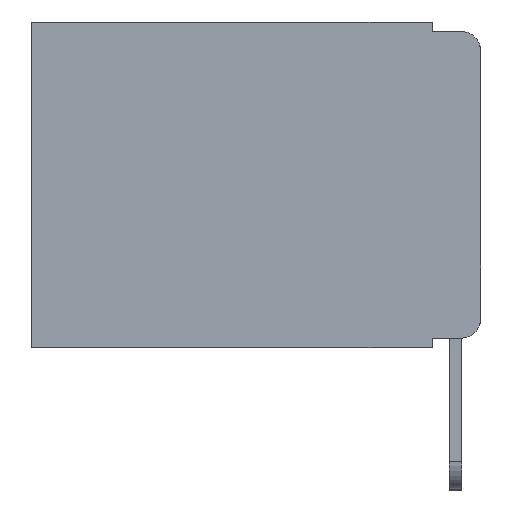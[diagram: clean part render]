
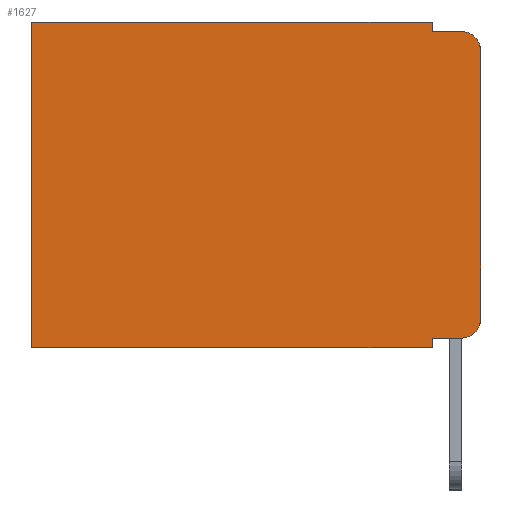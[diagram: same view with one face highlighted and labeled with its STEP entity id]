
A CAD part, left-side view. The second image highlights one B-rep face of the part: STEP entity #1627.
In plain terms, the highlighted planar face has unit normal (-1, 0, 0).
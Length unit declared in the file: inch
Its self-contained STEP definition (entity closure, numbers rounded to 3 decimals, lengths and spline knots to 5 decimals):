
#272 = CIRCLE ( 'NONE', #9551, 0.02 ) ;
#460 = VERTEX_POINT ( 'NONE', #11396 ) ;
#861 = VECTOR ( 'NONE', #10455, 39.37008 ) ;
#1310 = AXIS2_PLACEMENT_3D ( 'NONE', #9073, #3882, #10256 ) ;
#1342 = DIRECTION ( 'NONE',  ( 0., 1., 0. ) ) ;
#1490 = VECTOR ( 'NONE', #3290, 39.37008 ) ;
#1609 = EDGE_CURVE ( 'NONE', #9750, #5757, #6083, .T. ) ;
#1627 = ADVANCED_FACE ( 'NONE', ( #3625 ), #3471, .F. ) ;
#1780 = EDGE_CURVE ( 'NONE', #5310, #5757, #6770, .T. ) ;
#1840 = EDGE_CURVE ( 'NONE', #4678, #5310, #3176, .T. ) ;
#1926 = VERTEX_POINT ( 'NONE', #10651 ) ;
#2858 = VERTEX_POINT ( 'NONE', #3970 ) ;
#2883 = LINE ( 'NONE', #9524, #5368 ) ;
#3152 = DIRECTION ( 'NONE',  ( 0., 1., 0. ) ) ;
#3176 = LINE ( 'NONE', #5163, #7730 ) ;
#3192 = CARTESIAN_POINT ( 'NONE',  ( 0.298, 0.051, 0. ) ) ;
#3243 = EDGE_CURVE ( 'NONE', #6789, #460, #3718, .T. ) ;
#3264 = CARTESIAN_POINT ( 'NONE',  ( 0.298, 0.051, -0.01 ) ) ;
#3290 = DIRECTION ( 'NONE',  ( 0., 0., -1. ) ) ;
#3349 = DIRECTION ( 'NONE',  ( 1., 0., 0. ) ) ;
#3393 = DIRECTION ( 'NONE',  ( 0., 0., -1. ) ) ;
#3471 = PLANE ( 'NONE',  #3967 ) ;
#3625 = FACE_OUTER_BOUND ( 'NONE', #4723, .T. ) ;
#3718 = LINE ( 'NONE', #9774, #8160 ) ;
#3833 = VECTOR ( 'NONE', #3152, 39.37008 ) ;
#3861 = VERTEX_POINT ( 'NONE', #9793 ) ;
#3882 = DIRECTION ( 'NONE',  ( -1., 0., 0. ) ) ;
#3936 = CARTESIAN_POINT ( 'NONE',  ( 0.298, 0., 0. ) ) ;
#3967 = AXIS2_PLACEMENT_3D ( 'NONE', #7719, #3349, #3393 ) ;
#3970 = CARTESIAN_POINT ( 'NONE',  ( 0.298, 0.051, -0.333 ) ) ;
#4112 = LINE ( 'NONE', #5919, #3833 ) ;
#4230 = CARTESIAN_POINT ( 'NONE',  ( 0.298, 0.473, 0. ) ) ;
#4678 = VERTEX_POINT ( 'NONE', #3192 ) ;
#4723 = EDGE_LOOP ( 'NONE', ( #8483, #8191, #8712, #5086, #8840, #4931, #5181, #6356, #5758, #5106 ) ) ;
#4902 = DIRECTION ( 'NONE',  ( -1., 0., 0. ) ) ;
#4931 = ORIENTED_EDGE ( 'NONE', *, *, #9802, .T. ) ;
#5086 = ORIENTED_EDGE ( 'NONE', *, *, #1840, .F. ) ;
#5106 = ORIENTED_EDGE ( 'NONE', *, *, #8653, .T. ) ;
#5163 = CARTESIAN_POINT ( 'NONE',  ( 0.298, 0.051, 0. ) ) ;
#5181 = ORIENTED_EDGE ( 'NONE', *, *, #3243, .F. ) ;
#5310 = VERTEX_POINT ( 'NONE', #3264 ) ;
#5368 = VECTOR ( 'NONE', #10302, 39.37008 ) ;
#5757 = VERTEX_POINT ( 'NONE', #10799 ) ;
#5758 = ORIENTED_EDGE ( 'NONE', *, *, #11333, .T. ) ;
#5870 = CARTESIAN_POINT ( 'NONE',  ( 0.298, 0.051, -0.343 ) ) ;
#5919 = CARTESIAN_POINT ( 'NONE',  ( 0.298, 0., 0. ) ) ;
#6083 = CIRCLE ( 'NONE', #1310, 0.02 ) ;
#6356 = ORIENTED_EDGE ( 'NONE', *, *, #9963, .F. ) ;
#6399 = DIRECTION ( 'NONE',  ( 0., 0., -1. ) ) ;
#6403 = EDGE_CURVE ( 'NONE', #9750, #7958, #8564, .T. ) ;
#6770 = LINE ( 'NONE', #11725, #10818 ) ;
#6789 = VERTEX_POINT ( 'NONE', #5870 ) ;
#7719 = CARTESIAN_POINT ( 'NONE',  ( 0.298, 0., 0. ) ) ;
#7730 = VECTOR ( 'NONE', #6399, 39.37008 ) ;
#7958 = VERTEX_POINT ( 'NONE', #9181 ) ;
#8042 = EDGE_CURVE ( 'NONE', #4678, #3861, #4112, .T. ) ;
#8160 = VECTOR ( 'NONE', #1342, 39.37008 ) ;
#8191 = ORIENTED_EDGE ( 'NONE', *, *, #1609, .T. ) ;
#8483 = ORIENTED_EDGE ( 'NONE', *, *, #6403, .F. ) ;
#8564 = LINE ( 'NONE', #3936, #861 ) ;
#8653 = EDGE_CURVE ( 'NONE', #1926, #7958, #272, .T. ) ;
#8712 = ORIENTED_EDGE ( 'NONE', *, *, #1780, .F. ) ;
#8738 = LINE ( 'NONE', #4230, #1490 ) ;
#8840 = ORIENTED_EDGE ( 'NONE', *, *, #8042, .T. ) ;
#9073 = CARTESIAN_POINT ( 'NONE',  ( 0.298, 0.02, -0.03 ) ) ;
#9181 = CARTESIAN_POINT ( 'NONE',  ( 0.298, 0., -0.313 ) ) ;
#9302 = CARTESIAN_POINT ( 'NONE',  ( 0.298, 0., -0.03 ) ) ;
#9524 = CARTESIAN_POINT ( 'NONE',  ( 0.298, 0.051, -0.333 ) ) ;
#9551 = AXIS2_PLACEMENT_3D ( 'NONE', #9922, #4902, #10754 ) ;
#9750 = VERTEX_POINT ( 'NONE', #9302 ) ;
#9774 = CARTESIAN_POINT ( 'NONE',  ( 0.298, 0., -0.343 ) ) ;
#9793 = CARTESIAN_POINT ( 'NONE',  ( 0.298, 0.473, 0. ) ) ;
#9802 = EDGE_CURVE ( 'NONE', #3861, #460, #8738, .T. ) ;
#9922 = CARTESIAN_POINT ( 'NONE',  ( 0.298, 0.02, -0.313 ) ) ;
#9963 = EDGE_CURVE ( 'NONE', #2858, #6789, #11232, .T. ) ;
#10256 = DIRECTION ( 'NONE',  ( 0., 0., -1. ) ) ;
#10302 = DIRECTION ( 'NONE',  ( 0., -1., 0. ) ) ;
#10355 = CARTESIAN_POINT ( 'NONE',  ( 0.298, 0.051, 0. ) ) ;
#10455 = DIRECTION ( 'NONE',  ( 0., 0., -1. ) ) ;
#10651 = CARTESIAN_POINT ( 'NONE',  ( 0.298, 0.02, -0.333 ) ) ;
#10754 = DIRECTION ( 'NONE',  ( 0., 0., -1. ) ) ;
#10799 = CARTESIAN_POINT ( 'NONE',  ( 0.298, 0.02, -0.01 ) ) ;
#10818 = VECTOR ( 'NONE', #11739, 39.37008 ) ;
#10980 = VECTOR ( 'NONE', #11195, 39.37008 ) ;
#11195 = DIRECTION ( 'NONE',  ( 0., 0., -1. ) ) ;
#11232 = LINE ( 'NONE', #10355, #10980 ) ;
#11333 = EDGE_CURVE ( 'NONE', #2858, #1926, #2883, .T. ) ;
#11396 = CARTESIAN_POINT ( 'NONE',  ( 0.298, 0.473, -0.343 ) ) ;
#11725 = CARTESIAN_POINT ( 'NONE',  ( 0.298, 0.051, -0.01 ) ) ;
#11739 = DIRECTION ( 'NONE',  ( 0., -1., 0. ) ) ;
